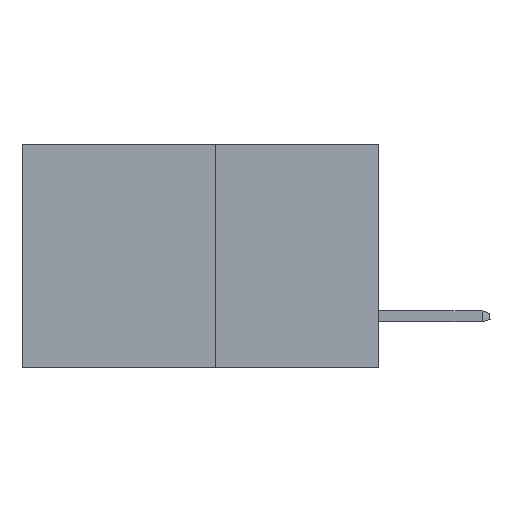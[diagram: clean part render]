
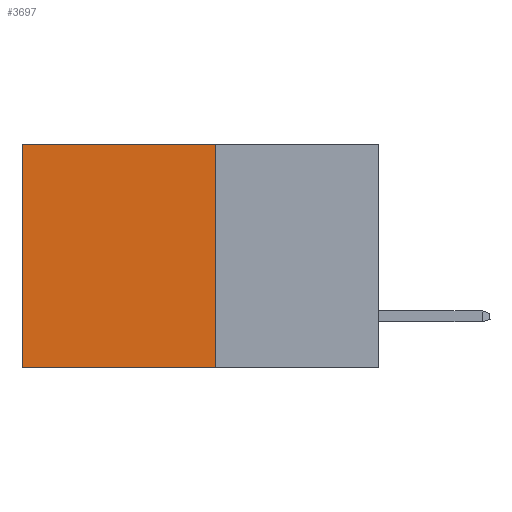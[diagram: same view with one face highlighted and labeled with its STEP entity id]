
A CAD part, left-side view. The second image highlights one B-rep face of the part: STEP entity #3697.
In plain terms, the highlighted planar face has unit normal (-1, 0, 0).
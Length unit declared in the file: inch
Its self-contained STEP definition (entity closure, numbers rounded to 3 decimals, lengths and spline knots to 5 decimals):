
#313 = LINE ( 'NONE', #10573, #3391 ) ;
#692 = CARTESIAN_POINT ( 'NONE',  ( 0.277, 0.27, 0. ) ) ;
#2126 = EDGE_CURVE ( 'NONE', #7980, #10544, #6766, .T. ) ;
#2142 = EDGE_CURVE ( 'NONE', #10544, #9016, #11423, .T. ) ;
#2182 = EDGE_CURVE ( 'NONE', #7980, #2547, #11284, .T. ) ;
#2377 = CARTESIAN_POINT ( 'NONE',  ( 0.277, 0.59, -0.37 ) ) ;
#2547 = VERTEX_POINT ( 'NONE', #8097 ) ;
#2615 = DIRECTION ( 'NONE',  ( 0., 1., 0. ) ) ;
#3391 = VECTOR ( 'NONE', #2615, 39.37008 ) ;
#3592 = DIRECTION ( 'NONE',  ( 0., 0., -1. ) ) ;
#3697 = ADVANCED_FACE ( 'NONE', ( #10563 ), #3860, .F. ) ;
#3745 = DIRECTION ( 'NONE',  ( 1., 0., 0. ) ) ;
#3782 = DIRECTION ( 'NONE',  ( 0., 1., 0. ) ) ;
#3860 = PLANE ( 'NONE',  #12476 ) ;
#5963 = EDGE_LOOP ( 'NONE', ( #8297, #6887, #6726, #9992 ) ) ;
#6308 = VECTOR ( 'NONE', #11537, 39.37008 ) ;
#6457 = VECTOR ( 'NONE', #3782, 39.37008 ) ;
#6726 = ORIENTED_EDGE ( 'NONE', *, *, #2182, .F. ) ;
#6766 = LINE ( 'NONE', #9235, #6457 ) ;
#6887 = ORIENTED_EDGE ( 'NONE', *, *, #9886, .F. ) ;
#7350 = CARTESIAN_POINT ( 'NONE',  ( 0.277, 0.27, -0.37 ) ) ;
#7579 = CARTESIAN_POINT ( 'NONE',  ( 0.277, 0.59, 0. ) ) ;
#7980 = VERTEX_POINT ( 'NONE', #692 ) ;
#8097 = CARTESIAN_POINT ( 'NONE',  ( 0.277, 0.27, -0.37 ) ) ;
#8297 = ORIENTED_EDGE ( 'NONE', *, *, #2142, .T. ) ;
#8960 = VECTOR ( 'NONE', #11574, 39.37008 ) ;
#9016 = VERTEX_POINT ( 'NONE', #2377 ) ;
#9235 = CARTESIAN_POINT ( 'NONE',  ( 0.277, 0.27, 0. ) ) ;
#9708 = CARTESIAN_POINT ( 'NONE',  ( 0.277, 0.27, -0.37 ) ) ;
#9886 = EDGE_CURVE ( 'NONE', #2547, #9016, #313, .T. ) ;
#9992 = ORIENTED_EDGE ( 'NONE', *, *, #2126, .T. ) ;
#10544 = VERTEX_POINT ( 'NONE', #7579 ) ;
#10563 = FACE_OUTER_BOUND ( 'NONE', #5963, .T. ) ;
#10573 = CARTESIAN_POINT ( 'NONE',  ( 0.277, 0.27, -0.37 ) ) ;
#11205 = CARTESIAN_POINT ( 'NONE',  ( 0.277, 0.59, -0.37 ) ) ;
#11284 = LINE ( 'NONE', #9708, #6308 ) ;
#11423 = LINE ( 'NONE', #11205, #8960 ) ;
#11537 = DIRECTION ( 'NONE',  ( 0., 0., -1. ) ) ;
#11574 = DIRECTION ( 'NONE',  ( 0., 0., -1. ) ) ;
#12476 = AXIS2_PLACEMENT_3D ( 'NONE', #7350, #3745, #3592 ) ;
